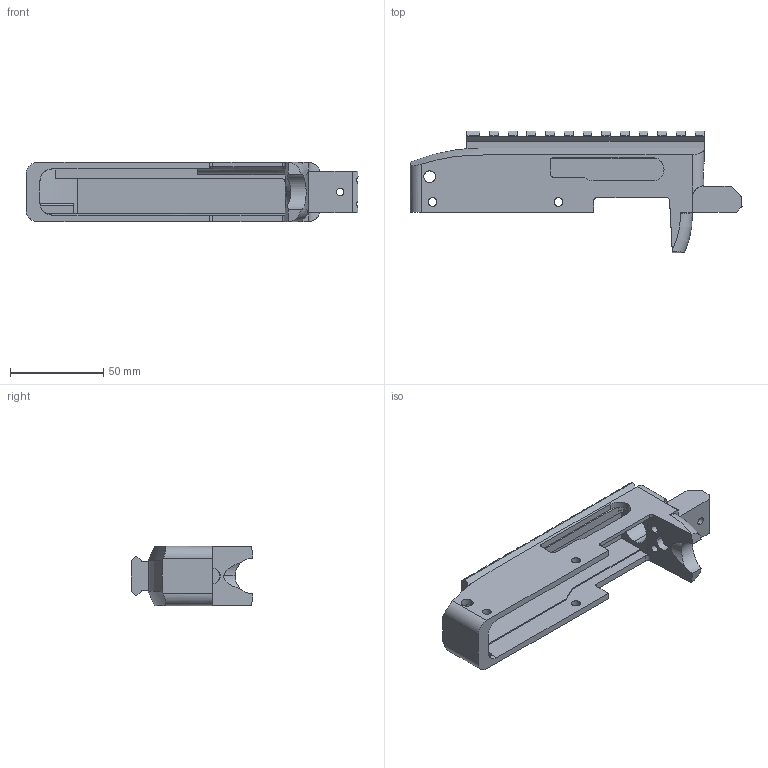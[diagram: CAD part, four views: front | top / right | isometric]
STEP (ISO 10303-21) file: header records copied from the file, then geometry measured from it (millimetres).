
FILE_DESCRIPTION (( 'STEP AP214' ), '1' );
FILE_NAME ('10-22.STEP', '2014-07-09T16:35:08', ( 'WarFairy' ), ( '' ), 'SwSTEP 2.0', 'SolidWorks 2013', '' );
FILE_SCHEMA (( 'AUTOMOTIVE_DESIGN' ));
Length unit declared in the file: millimetre
Products named in the file (1): 10-22
Bounding box: 177.8 x 65.25 x 31.75 mm (x, y, z)
Volume: 83317.6 mm3; surface area: 37987 mm2
Topology: 1 solids, 1 shells, 210 faces, 633 edges, 420 vertices
Faces by surface type: plane 138, cylinder 63, bspline 5, torus 4
Entity records: 8361 total; most frequent: CARTESIAN_POINT 2676, ORIENTED_EDGE 1262, DIRECTION 1079, EDGE_CURVE 631, VECTOR 451, LINE 451, VERTEX_POINT 420, AXIS2_PLACEMENT_3D 314
